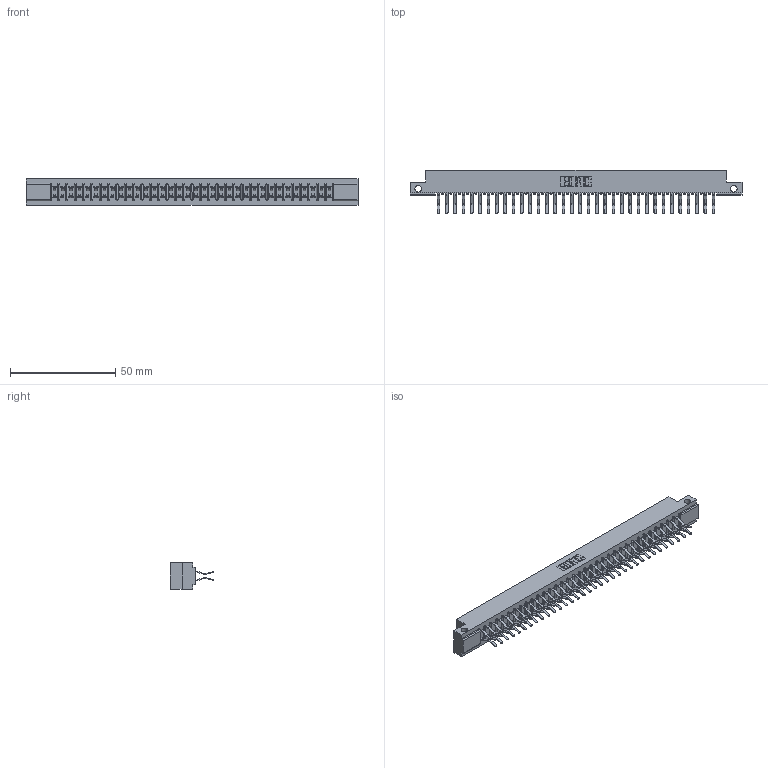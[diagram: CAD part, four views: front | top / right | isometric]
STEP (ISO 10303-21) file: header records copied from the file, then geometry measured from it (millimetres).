
FILE_DESCRIPTION (( 'STEP AP203' ), '1' );
FILE_NAME ('357-068-460-212.STEP', '2020-10-04T22:54:19', ( '' ), ( '' ), 'SwSTEP 2.0', 'SolidWorks 2020', '' );
FILE_SCHEMA (( 'CONFIG_CONTROL_DESIGN' ));
Length unit declared in the file: inch
Products named in the file (3): 307 Part_.128 Dia Side Mounting Holes; 357-068-460-212; 307-290-001_560
Assembly tree (69 placements, depth 2):
  357-068-460-212
    307 Part_.128 Dia Side Mounting Holes
    307-290-001_560  x68
Bounding box: 157.73 x 20.73 x 12.7 mm (x, y, z)
Volume: 16659.1 mm3; surface area: 20663.7 mm2
Topology: 69 solids, 69 shells, 3553 faces, 9979 edges, 6466 vertices
Faces by surface type: plane 2314, cylinder 1169, sphere 70
Entity records: 31328 total; most frequent: CARTESIAN_POINT 5126, ORIENTED_EDGE 5078, DIRECTION 5025, EDGE_CURVE 2539, LINE 1943, VECTOR 1943, VERTEX_POINT 1642, AXIS2_PLACEMENT_3D 1541
